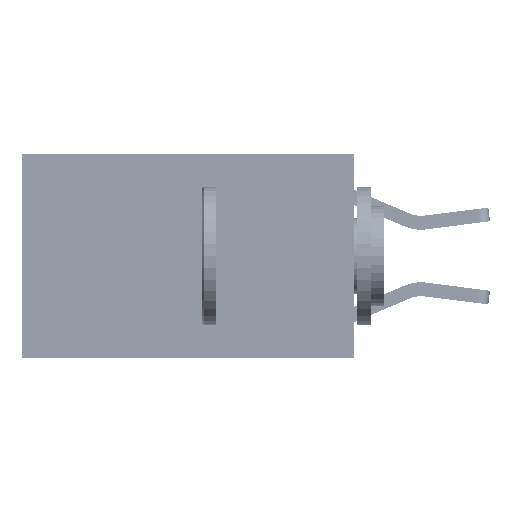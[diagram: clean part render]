
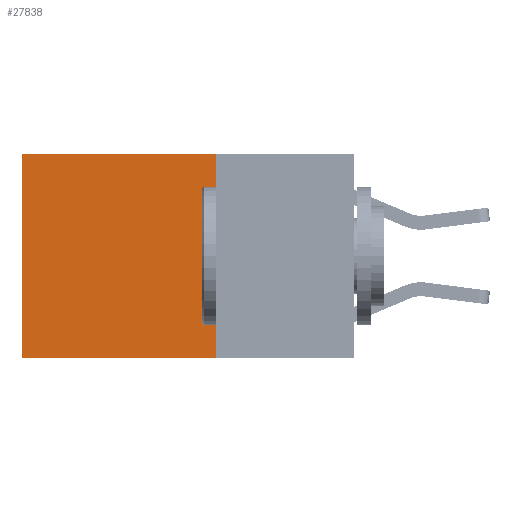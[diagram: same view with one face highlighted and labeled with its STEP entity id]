
A CAD part, left-side view. The second image highlights one B-rep face of the part: STEP entity #27838.
In plain terms, the highlighted planar face has unit normal (-1, 0, 0).
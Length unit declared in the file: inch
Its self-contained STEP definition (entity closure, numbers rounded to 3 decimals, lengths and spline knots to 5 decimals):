
#681 = DIRECTION ( 'NONE',  ( 0., 0., -1. ) ) ;
#823 = DIRECTION ( 'NONE',  ( 0., 1., 0. ) ) ;
#1708 = VECTOR ( 'NONE', #22305, 39.37008 ) ;
#2307 = EDGE_LOOP ( 'NONE', ( #2910, #17871, #11371, #18230 ) ) ;
#2497 = EDGE_CURVE ( 'NONE', #29807, #2949, #16461, .T. ) ;
#2910 = ORIENTED_EDGE ( 'NONE', *, *, #2497, .T. ) ;
#2949 = VERTEX_POINT ( 'NONE', #6903 ) ;
#3298 = LINE ( 'NONE', #29780, #1708 ) ;
#6903 = CARTESIAN_POINT ( 'NONE',  ( 0.2625, 0.6, -0.37 ) ) ;
#7032 = FACE_OUTER_BOUND ( 'NONE', #2307, .T. ) ;
#8358 = VECTOR ( 'NONE', #27499, 39.37008 ) ;
#11371 = ORIENTED_EDGE ( 'NONE', *, *, #31325, .F. ) ;
#12678 = LINE ( 'NONE', #28443, #25179 ) ;
#13271 = PLANE ( 'NONE',  #22268 ) ;
#15660 = VECTOR ( 'NONE', #17869, 39.37008 ) ;
#15758 = DIRECTION ( 'NONE',  ( 1., 0., 0. ) ) ;
#16461 = LINE ( 'NONE', #27896, #15660 ) ;
#17869 = DIRECTION ( 'NONE',  ( 0., 0., -1. ) ) ;
#17871 = ORIENTED_EDGE ( 'NONE', *, *, #20175, .F. ) ;
#18230 = ORIENTED_EDGE ( 'NONE', *, *, #24948, .T. ) ;
#20175 = EDGE_CURVE ( 'NONE', #27961, #2949, #12678, .T. ) ;
#20574 = VERTEX_POINT ( 'NONE', #27295 ) ;
#22268 = AXIS2_PLACEMENT_3D ( 'NONE', #28304, #15758, #681 ) ;
#22305 = DIRECTION ( 'NONE',  ( 0., 0., -1. ) ) ;
#23256 = LINE ( 'NONE', #24920, #8358 ) ;
#24920 = CARTESIAN_POINT ( 'NONE',  ( 0.2625, 0.25, 0. ) ) ;
#24948 = EDGE_CURVE ( 'NONE', #20574, #29807, #23256, .T. ) ;
#25179 = VECTOR ( 'NONE', #823, 39.37008 ) ;
#26293 = CARTESIAN_POINT ( 'NONE',  ( 0.2625, 0.25, -0.37 ) ) ;
#27295 = CARTESIAN_POINT ( 'NONE',  ( 0.2625, 0.25, 0. ) ) ;
#27499 = DIRECTION ( 'NONE',  ( 0., 1., 0. ) ) ;
#27838 = ADVANCED_FACE ( 'NONE', ( #7032 ), #13271, .F. ) ;
#27896 = CARTESIAN_POINT ( 'NONE',  ( 0.2625, 0.6, 0. ) ) ;
#27961 = VERTEX_POINT ( 'NONE', #26293 ) ;
#28304 = CARTESIAN_POINT ( 'NONE',  ( 0.2625, 0.25, 0. ) ) ;
#28426 = CARTESIAN_POINT ( 'NONE',  ( 0.2625, 0.6, 0. ) ) ;
#28443 = CARTESIAN_POINT ( 'NONE',  ( 0.2625, 0.25, -0.37 ) ) ;
#29780 = CARTESIAN_POINT ( 'NONE',  ( 0.2625, 0.25, 0. ) ) ;
#29807 = VERTEX_POINT ( 'NONE', #28426 ) ;
#31325 = EDGE_CURVE ( 'NONE', #20574, #27961, #3298, .T. ) ;
